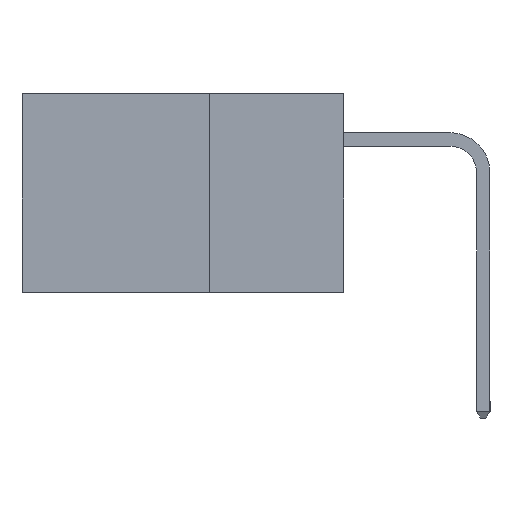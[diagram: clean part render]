
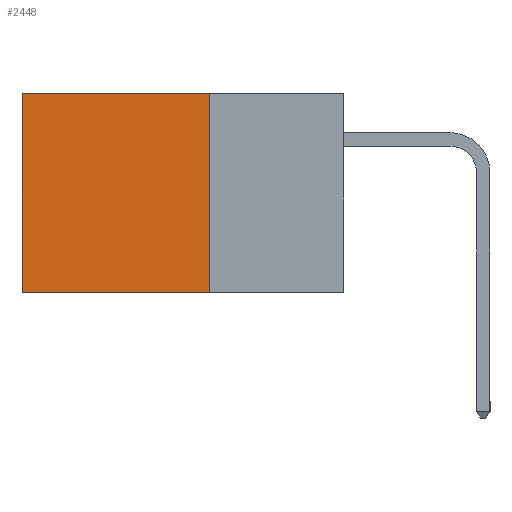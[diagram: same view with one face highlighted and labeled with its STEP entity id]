
A CAD part, left-side view. The second image highlights one B-rep face of the part: STEP entity #2448.
In plain terms, the highlighted planar face has unit normal (-1, 0, 0).
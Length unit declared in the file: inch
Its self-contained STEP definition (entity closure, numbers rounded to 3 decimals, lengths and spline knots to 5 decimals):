
#1648 = EDGE_LOOP ( 'NONE', ( #9598, #3436, #15669, #11701 ) ) ;
#2448 = ADVANCED_FACE ( 'NONE', ( #6945 ), #9525, .F. ) ;
#2855 = CARTESIAN_POINT ( 'NONE',  ( 0.2615, 0.25, -0.37 ) ) ;
#3247 = LINE ( 'NONE', #13438, #7749 ) ;
#3436 = ORIENTED_EDGE ( 'NONE', *, *, #10409, .F. ) ;
#3975 = EDGE_CURVE ( 'NONE', #22281, #10244, #3247, .T. ) ;
#4277 = AXIS2_PLACEMENT_3D ( 'NONE', #2855, #9502, #9397 ) ;
#6845 = VECTOR ( 'NONE', #18829, 39.37008 ) ;
#6945 = FACE_OUTER_BOUND ( 'NONE', #1648, .T. ) ;
#7749 = VECTOR ( 'NONE', #13208, 39.37008 ) ;
#8318 = EDGE_CURVE ( 'NONE', #10244, #15573, #10775, .T. ) ;
#9397 = DIRECTION ( 'NONE',  ( 0., 0., -1. ) ) ;
#9502 = DIRECTION ( 'NONE',  ( 1., 0., 0. ) ) ;
#9525 = PLANE ( 'NONE',  #4277 ) ;
#9598 = ORIENTED_EDGE ( 'NONE', *, *, #8318, .T. ) ;
#10186 = VECTOR ( 'NONE', #14832, 39.37008 ) ;
#10244 = VERTEX_POINT ( 'NONE', #20144 ) ;
#10409 = EDGE_CURVE ( 'NONE', #17093, #15573, #21178, .T. ) ;
#10775 = LINE ( 'NONE', #10797, #10186 ) ;
#10797 = CARTESIAN_POINT ( 'NONE',  ( 0.2615, 0.6, -0.37 ) ) ;
#11701 = ORIENTED_EDGE ( 'NONE', *, *, #3975, .T. ) ;
#13208 = DIRECTION ( 'NONE',  ( 0., 1., 0. ) ) ;
#13438 = CARTESIAN_POINT ( 'NONE',  ( 0.2615, 0.25, 0. ) ) ;
#14254 = CARTESIAN_POINT ( 'NONE',  ( 0.2615, 0.25, -0.37 ) ) ;
#14771 = LINE ( 'NONE', #22508, #19171 ) ;
#14832 = DIRECTION ( 'NONE',  ( 0., 0., -1. ) ) ;
#15573 = VERTEX_POINT ( 'NONE', #21612 ) ;
#15669 = ORIENTED_EDGE ( 'NONE', *, *, #22345, .F. ) ;
#16763 = DIRECTION ( 'NONE',  ( 0., 0., -1. ) ) ;
#17093 = VERTEX_POINT ( 'NONE', #14254 ) ;
#18829 = DIRECTION ( 'NONE',  ( 0., 1., 0. ) ) ;
#19095 = CARTESIAN_POINT ( 'NONE',  ( 0.2615, 0.25, -0.37 ) ) ;
#19171 = VECTOR ( 'NONE', #16763, 39.37008 ) ;
#20144 = CARTESIAN_POINT ( 'NONE',  ( 0.2615, 0.6, 0. ) ) ;
#21178 = LINE ( 'NONE', #19095, #6845 ) ;
#21612 = CARTESIAN_POINT ( 'NONE',  ( 0.2615, 0.6, -0.37 ) ) ;
#22281 = VERTEX_POINT ( 'NONE', #22342 ) ;
#22342 = CARTESIAN_POINT ( 'NONE',  ( 0.2615, 0.25, 0. ) ) ;
#22345 = EDGE_CURVE ( 'NONE', #22281, #17093, #14771, .T. ) ;
#22508 = CARTESIAN_POINT ( 'NONE',  ( 0.2615, 0.25, -0.37 ) ) ;
